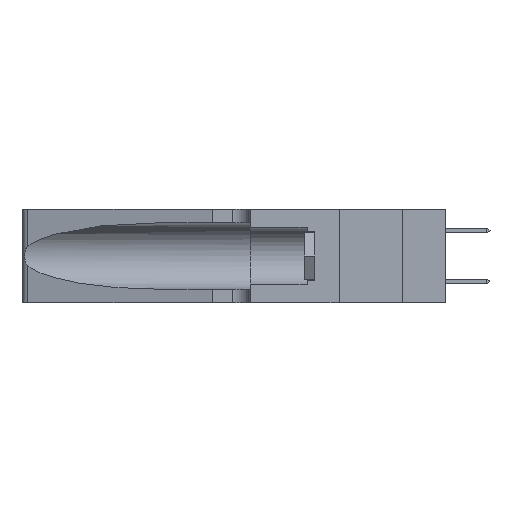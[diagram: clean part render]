
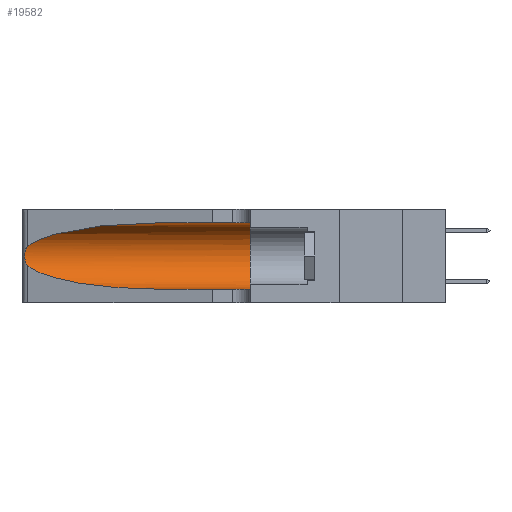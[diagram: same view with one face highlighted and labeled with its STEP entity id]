
A CAD part, left-side view. The second image highlights one B-rep face of the part: STEP entity #19582.
In plain terms, the highlighted cylindrical face has radius 3.308 mm (diameter 6.617 mm), a partial arc.
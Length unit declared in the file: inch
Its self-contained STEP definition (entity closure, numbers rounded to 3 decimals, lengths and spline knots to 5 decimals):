
#169 = EDGE_CURVE ( 'NONE', #15435, #13026, #14288, .T. ) ;
#573 = ORIENTED_EDGE ( 'NONE', *, *, #4456, .T. ) ;
#896 = CARTESIAN_POINT ( 'NONE',  ( 0.25487, 1.22718, 0.14631 ) ) ;
#1204 = DIRECTION ( 'NONE',  ( 0., -1., 0. ) ) ;
#1527 = ORIENTED_EDGE ( 'NONE', *, *, #169, .F. ) ;
#1748 =( BOUNDED_CURVE ( )  B_SPLINE_CURVE ( 3, ( #18619, #18536, #12932, #20372 ),
 .UNSPECIFIED., .F., .F. ) 
 B_SPLINE_CURVE_WITH_KNOTS ( ( 4, 4 ),
 ( 1.5708, 2.84003 ),
 .UNSPECIFIED. ) 
 CURVE ( )  GEOMETRIC_REPRESENTATION_ITEM ( )  RATIONAL_B_SPLINE_CURVE ( ( 1., 0.87, 0.87, 1. ) ) 
 REPRESENTATION_ITEM ( '' )  );
#2140 = CARTESIAN_POINT ( 'NONE',  ( 0.1305, 0.72297, 0.31525 ) ) ;
#2200 = B_SPLINE_CURVE_WITH_KNOTS ( 'NONE', 3,
 ( #16836, #9266, #5650, #24289, #3449, #7226, #20719, #24056, #13045, #14937, #3690, #20409, #22260, #10999 ),
 .UNSPECIFIED., .F., .F.,
 ( 4, 2, 2, 2, 2, 2, 4 ),
 ( 0., 0.00027, 0.00053, 0.00107, 0.0016, 0.00187, 0.00214 ),
 .UNSPECIFIED. ) ;
#2337 = CARTESIAN_POINT ( 'NONE',  ( 0.1305, 0.35, 0.31525 ) ) ;
#2378 = CARTESIAN_POINT ( 'NONE',  ( 0.1305, 1.61858, 0.05475 ) ) ;
#3449 = CARTESIAN_POINT ( 'NONE',  ( 0.25854, 1.2359, 0.20912 ) ) ;
#3690 = CARTESIAN_POINT ( 'NONE',  ( 0.25789, 1.23486, 0.15765 ) ) ;
#3966 = ORIENTED_EDGE ( 'NONE', *, *, #8517, .T. ) ;
#4456 = EDGE_CURVE ( 'NONE', #13320, #5963, #2200, .T. ) ;
#4862 = EDGE_CURVE ( 'NONE', #13026, #20568, #19762, .T. ) ;
#5110 = CARTESIAN_POINT ( 'NONE',  ( 0.1305, 0.35, 0.185 ) ) ;
#5541 = CYLINDRICAL_SURFACE ( 'NONE', #15214, 0.13025 ) ;
#5650 = CARTESIAN_POINT ( 'NONE',  ( 0.25639, 1.23184, 0.21858 ) ) ;
#5834 = ORIENTED_EDGE ( 'NONE', *, *, #10597, .T. ) ;
#5963 = VERTEX_POINT ( 'NONE', #896 ) ;
#6027 = LINE ( 'NONE', #2378, #13656 ) ;
#6089 = DIRECTION ( 'NONE',  ( 0., -1., 0. ) ) ;
#6112 = AXIS2_PLACEMENT_3D ( 'NONE', #5110, #20332, #8869 ) ;
#7226 = CARTESIAN_POINT ( 'NONE',  ( 0.26018, 1.23835, 0.19895 ) ) ;
#7340 = CARTESIAN_POINT ( 'NONE',  ( 0.25487, 1.22718, 0.14631 ) ) ;
#8090 = CARTESIAN_POINT ( 'NONE',  ( 0.1305, 0.35, 0.05475 ) ) ;
#8139 = ORIENTED_EDGE ( 'NONE', *, *, #9794, .T. ) ;
#8517 = EDGE_CURVE ( 'NONE', #16802, #20568, #6027, .T. ) ;
#8869 = DIRECTION ( 'NONE',  ( 0., 0., 1. ) ) ;
#9266 = CARTESIAN_POINT ( 'NONE',  ( 0.25555, 1.22994, 0.2215 ) ) ;
#9794 = EDGE_CURVE ( 'NONE', #5963, #16802, #17110, .T. ) ;
#10597 = EDGE_CURVE ( 'NONE', #15435, #13320, #1748, .T. ) ;
#10682 = DIRECTION ( 'NONE',  ( 0., -1., 0. ) ) ;
#10769 = EDGE_LOOP ( 'NONE', ( #5834, #573, #8139, #3966, #15550, #1527 ) ) ;
#10999 = CARTESIAN_POINT ( 'NONE',  ( 0.25487, 1.22718, 0.14631 ) ) ;
#11114 = CARTESIAN_POINT ( 'NONE',  ( 0.18966, 0.96281, 0.05475 ) ) ;
#12493 = CARTESIAN_POINT ( 'NONE',  ( 0.1305, 1.61858, 0.185 ) ) ;
#12932 = CARTESIAN_POINT ( 'NONE',  ( 0.2373, 1.15595, 0.28018 ) ) ;
#13026 = VERTEX_POINT ( 'NONE', #2337 ) ;
#13045 = CARTESIAN_POINT ( 'NONE',  ( 0.26017, 1.23833, 0.17102 ) ) ;
#13320 = VERTEX_POINT ( 'NONE', #20579 ) ;
#13359 = CARTESIAN_POINT ( 'NONE',  ( 0.1305, 0.72297, 0.05475 ) ) ;
#13656 = VECTOR ( 'NONE', #6089, 39.37008 ) ;
#14288 = LINE ( 'NONE', #16266, #22223 ) ;
#14298 = DIRECTION ( 'NONE',  ( 0., 0., -1. ) ) ;
#14365 = FACE_OUTER_BOUND ( 'NONE', #10769, .T. ) ;
#14937 = CARTESIAN_POINT ( 'NONE',  ( 0.25856, 1.23593, 0.16098 ) ) ;
#15214 = AXIS2_PLACEMENT_3D ( 'NONE', #12493, #1204, #14298 ) ;
#15435 = VERTEX_POINT ( 'NONE', #2140 ) ;
#15550 = ORIENTED_EDGE ( 'NONE', *, *, #4862, .F. ) ;
#16266 = CARTESIAN_POINT ( 'NONE',  ( 0.1305, 1.61858, 0.31525 ) ) ;
#16802 = VERTEX_POINT ( 'NONE', #13359 ) ;
#16836 = CARTESIAN_POINT ( 'NONE',  ( 0.25487, 1.22718, 0.22369 ) ) ;
#17110 =( BOUNDED_CURVE ( )  B_SPLINE_CURVE ( 3, ( #7340, #20515, #11114, #20440 ),
 .UNSPECIFIED., .F., .T. ) 
 B_SPLINE_CURVE_WITH_KNOTS ( ( 4, 4 ),
 ( 3.44316, 4.71239 ),
 .UNSPECIFIED. ) 
 CURVE ( )  GEOMETRIC_REPRESENTATION_ITEM ( )  RATIONAL_B_SPLINE_CURVE ( ( 1., 0.87, 0.87, 1. ) ) 
 REPRESENTATION_ITEM ( '' )  );
#18536 = CARTESIAN_POINT ( 'NONE',  ( 0.18966, 0.96281, 0.31525 ) ) ;
#18619 = CARTESIAN_POINT ( 'NONE',  ( 0.1305, 0.72297, 0.31525 ) ) ;
#19582 = ADVANCED_FACE ( 'NONE', ( #14365 ), #5541, .F. ) ;
#19762 = CIRCLE ( 'NONE', #6112, 0.13025 ) ;
#20332 = DIRECTION ( 'NONE',  ( 0., 1., 0. ) ) ;
#20372 = CARTESIAN_POINT ( 'NONE',  ( 0.25487, 1.22718, 0.22369 ) ) ;
#20409 = CARTESIAN_POINT ( 'NONE',  ( 0.25639, 1.23186, 0.15144 ) ) ;
#20440 = CARTESIAN_POINT ( 'NONE',  ( 0.1305, 0.72297, 0.05475 ) ) ;
#20515 = CARTESIAN_POINT ( 'NONE',  ( 0.2373, 1.15595, 0.08982 ) ) ;
#20568 = VERTEX_POINT ( 'NONE', #8090 ) ;
#20579 = CARTESIAN_POINT ( 'NONE',  ( 0.25487, 1.22718, 0.22369 ) ) ;
#20719 = CARTESIAN_POINT ( 'NONE',  ( 0.26075, 1.23896, 0.19203 ) ) ;
#22223 = VECTOR ( 'NONE', #10682, 39.37008 ) ;
#22260 = CARTESIAN_POINT ( 'NONE',  ( 0.25555, 1.22993, 0.14849 ) ) ;
#24056 = CARTESIAN_POINT ( 'NONE',  ( 0.26075, 1.23896, 0.178 ) ) ;
#24289 = CARTESIAN_POINT ( 'NONE',  ( 0.25787, 1.23484, 0.2124 ) ) ;
